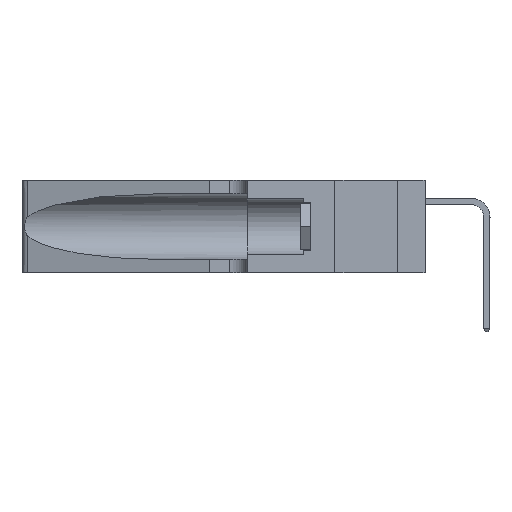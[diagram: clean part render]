
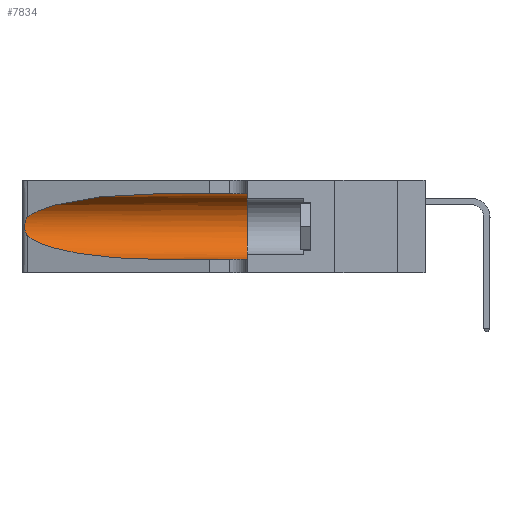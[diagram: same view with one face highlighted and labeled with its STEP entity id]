
A CAD part, left-side view. The second image highlights one B-rep face of the part: STEP entity #7834.
In plain terms, the highlighted cylindrical face has radius 3.308 mm (diameter 6.617 mm), a partial arc.
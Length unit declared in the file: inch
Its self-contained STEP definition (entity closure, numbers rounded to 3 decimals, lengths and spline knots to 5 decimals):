
#302 = CARTESIAN_POINT ( 'NONE',  ( 0.1305, 1.61858, 0.31525 ) ) ;
#685 = CARTESIAN_POINT ( 'NONE',  ( 0.1305, 1.61858, 0.185 ) ) ;
#1232 = DIRECTION ( 'NONE',  ( 0., -1., 0. ) ) ;
#1372 = CARTESIAN_POINT ( 'NONE',  ( 0.25487, 1.22718, 0.22369 ) ) ;
#1446 = ORIENTED_EDGE ( 'NONE', *, *, #23722, .T. ) ;
#1892 = ORIENTED_EDGE ( 'NONE', *, *, #7507, .F. ) ;
#2685 = VECTOR ( 'NONE', #18355, 39.37008 ) ;
#2760 = CARTESIAN_POINT ( 'NONE',  ( 0.2373, 1.15595, 0.08982 ) ) ;
#2946 = CARTESIAN_POINT ( 'NONE',  ( 0.26075, 1.23896, 0.178 ) ) ;
#3511 = B_SPLINE_CURVE_WITH_KNOTS ( 'NONE', 3,
 ( #29678, #35409, #14983, #35542, #17936, #38482, #20941, #2946, #23907, #6003, #26860, #9062, #29810, #12112 ),
 .UNSPECIFIED., .F., .F.,
 ( 4, 2, 2, 2, 2, 2, 4 ),
 ( 0., 0.00027, 0.00053, 0.00107, 0.0016, 0.00187, 0.00214 ),
 .UNSPECIFIED. ) ;
#4841 = VERTEX_POINT ( 'NONE', #20879 ) ;
#5595 = LINE ( 'NONE', #36829, #36206 ) ;
#5779 = VERTEX_POINT ( 'NONE', #1372 ) ;
#5815 = CARTESIAN_POINT ( 'NONE',  ( 0.25487, 1.22718, 0.14631 ) ) ;
#5892 = ORIENTED_EDGE ( 'NONE', *, *, #12609, .T. ) ;
#6003 = CARTESIAN_POINT ( 'NONE',  ( 0.25856, 1.23593, 0.16098 ) ) ;
#7507 = EDGE_CURVE ( 'NONE', #10291, #12182, #15053, .T. ) ;
#7834 = ADVANCED_FACE ( 'NONE', ( #9860 ), #23820, .F. ) ;
#8556 = EDGE_LOOP ( 'NONE', ( #11201, #11674, #5892, #1446, #1892, #20362 ) ) ;
#8876 = CARTESIAN_POINT ( 'NONE',  ( 0.18966, 0.96281, 0.05475 ) ) ;
#9062 = CARTESIAN_POINT ( 'NONE',  ( 0.25639, 1.23186, 0.15144 ) ) ;
#9860 = FACE_OUTER_BOUND ( 'NONE', #8556, .T. ) ;
#10291 = VERTEX_POINT ( 'NONE', #18177 ) ;
#10614 = CARTESIAN_POINT ( 'NONE',  ( 0.1305, 0.72297, 0.05475 ) ) ;
#10773 = LINE ( 'NONE', #302, #2685 ) ;
#10941 = CARTESIAN_POINT ( 'NONE',  ( 0.2373, 1.15595, 0.28018 ) ) ;
#11201 = ORIENTED_EDGE ( 'NONE', *, *, #26486, .T. ) ;
#11213 = CARTESIAN_POINT ( 'NONE',  ( 0.1305, 0.35, 0.185 ) ) ;
#11674 = ORIENTED_EDGE ( 'NONE', *, *, #12013, .T. ) ;
#12013 = EDGE_CURVE ( 'NONE', #5779, #24905, #3511, .T. ) ;
#12112 = CARTESIAN_POINT ( 'NONE',  ( 0.25487, 1.22718, 0.14631 ) ) ;
#12182 = VERTEX_POINT ( 'NONE', #21847 ) ;
#12609 = EDGE_CURVE ( 'NONE', #24905, #22505, #30291, .T. ) ;
#12644 = CARTESIAN_POINT ( 'NONE',  ( 0.25487, 1.22718, 0.14631 ) ) ;
#13929 =( BOUNDED_CURVE ( )  B_SPLINE_CURVE ( 3, ( #25736, #28679, #10941, #31646 ),
 .UNSPECIFIED., .F., .F. ) 
 B_SPLINE_CURVE_WITH_KNOTS ( ( 4, 4 ),
 ( 1.5708, 2.84003 ),
 .UNSPECIFIED. ) 
 CURVE ( )  GEOMETRIC_REPRESENTATION_ITEM ( )  RATIONAL_B_SPLINE_CURVE ( ( 1., 0.87, 0.87, 1. ) ) 
 REPRESENTATION_ITEM ( '' )  );
#14248 = DIRECTION ( 'NONE',  ( 0., 0., 1. ) ) ;
#14983 = CARTESIAN_POINT ( 'NONE',  ( 0.25639, 1.23184, 0.21858 ) ) ;
#15053 = CIRCLE ( 'NONE', #25479, 0.13025 ) ;
#17936 = CARTESIAN_POINT ( 'NONE',  ( 0.25854, 1.2359, 0.20912 ) ) ;
#18177 = CARTESIAN_POINT ( 'NONE',  ( 0.1305, 0.35, 0.31525 ) ) ;
#18355 = DIRECTION ( 'NONE',  ( 0., -1., 0. ) ) ;
#18583 = DIRECTION ( 'NONE',  ( 0., -1., 0. ) ) ;
#20362 = ORIENTED_EDGE ( 'NONE', *, *, #26195, .F. ) ;
#20879 = CARTESIAN_POINT ( 'NONE',  ( 0.1305, 0.72297, 0.31525 ) ) ;
#20941 = CARTESIAN_POINT ( 'NONE',  ( 0.26075, 1.23896, 0.19203 ) ) ;
#21847 = CARTESIAN_POINT ( 'NONE',  ( 0.1305, 0.35, 0.05475 ) ) ;
#22505 = VERTEX_POINT ( 'NONE', #10614 ) ;
#23722 = EDGE_CURVE ( 'NONE', #22505, #12182, #5595, .T. ) ;
#23820 = CYLINDRICAL_SURFACE ( 'NONE', #32599, 0.13025 ) ;
#23907 = CARTESIAN_POINT ( 'NONE',  ( 0.26017, 1.23833, 0.17102 ) ) ;
#24905 = VERTEX_POINT ( 'NONE', #12644 ) ;
#25479 = AXIS2_PLACEMENT_3D ( 'NONE', #11213, #31909, #14248 ) ;
#25736 = CARTESIAN_POINT ( 'NONE',  ( 0.1305, 0.72297, 0.31525 ) ) ;
#26195 = EDGE_CURVE ( 'NONE', #4841, #10291, #10773, .T. ) ;
#26486 = EDGE_CURVE ( 'NONE', #4841, #5779, #13929, .T. ) ;
#26860 = CARTESIAN_POINT ( 'NONE',  ( 0.25789, 1.23486, 0.15765 ) ) ;
#28679 = CARTESIAN_POINT ( 'NONE',  ( 0.18966, 0.96281, 0.31525 ) ) ;
#29632 = CARTESIAN_POINT ( 'NONE',  ( 0.1305, 0.72297, 0.05475 ) ) ;
#29678 = CARTESIAN_POINT ( 'NONE',  ( 0.25487, 1.22718, 0.22369 ) ) ;
#29810 = CARTESIAN_POINT ( 'NONE',  ( 0.25555, 1.22993, 0.14849 ) ) ;
#30291 =( BOUNDED_CURVE ( )  B_SPLINE_CURVE ( 3, ( #5815, #2760, #8876, #29632 ),
 .UNSPECIFIED., .F., .F. ) 
 B_SPLINE_CURVE_WITH_KNOTS ( ( 4, 4 ),
 ( 3.44316, 4.71239 ),
 .UNSPECIFIED. ) 
 CURVE ( )  GEOMETRIC_REPRESENTATION_ITEM ( )  RATIONAL_B_SPLINE_CURVE ( ( 1., 0.87, 0.87, 1. ) ) 
 REPRESENTATION_ITEM ( '' )  );
#30475 = DIRECTION ( 'NONE',  ( 0., 0., -1. ) ) ;
#31646 = CARTESIAN_POINT ( 'NONE',  ( 0.25487, 1.22718, 0.22369 ) ) ;
#31909 = DIRECTION ( 'NONE',  ( 0., 1., 0. ) ) ;
#32599 = AXIS2_PLACEMENT_3D ( 'NONE', #685, #18583, #30475 ) ;
#35409 = CARTESIAN_POINT ( 'NONE',  ( 0.25555, 1.22994, 0.2215 ) ) ;
#35542 = CARTESIAN_POINT ( 'NONE',  ( 0.25787, 1.23484, 0.2124 ) ) ;
#36206 = VECTOR ( 'NONE', #1232, 39.37008 ) ;
#36829 = CARTESIAN_POINT ( 'NONE',  ( 0.1305, 1.61858, 0.05475 ) ) ;
#38482 = CARTESIAN_POINT ( 'NONE',  ( 0.26018, 1.23835, 0.19895 ) ) ;
